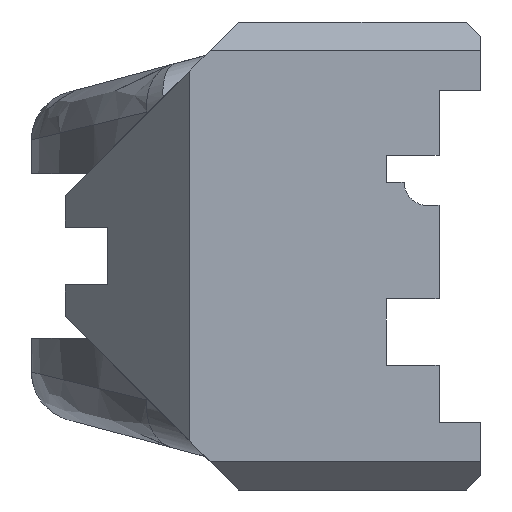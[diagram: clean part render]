
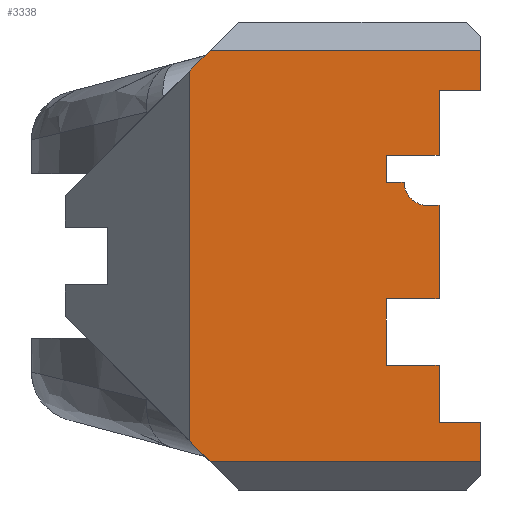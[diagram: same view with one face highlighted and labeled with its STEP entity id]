
A CAD part, left-side view. The second image highlights one B-rep face of the part: STEP entity #3338.
In plain terms, the highlighted planar face has unit normal (-1, 0, 0).
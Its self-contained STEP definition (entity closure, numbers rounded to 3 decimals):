
#82=PLANE('',#3544);
#240=FACE_OUTER_BOUND('',#420,.T.);
#420=EDGE_LOOP('',(#2469,#2470,#2471,#2472,#2473,#2474,#2475,#2476,#2477,
#2478,#2479,#2480,#2481,#2482,#2483,#2484,#2485,#2486,#2487,#2488));
#700=LINE('',#4953,#1138);
#701=LINE('',#4955,#1139);
#702=LINE('',#4957,#1140);
#703=LINE('',#4959,#1141);
#704=LINE('',#4961,#1142);
#705=LINE('',#4963,#1143);
#706=LINE('',#4965,#1144);
#707=LINE('',#4967,#1145);
#708=LINE('',#4969,#1146);
#709=LINE('',#4971,#1147);
#710=LINE('',#4973,#1148);
#711=LINE('',#4975,#1149);
#712=LINE('',#4979,#1150);
#713=LINE('',#4981,#1151);
#714=LINE('',#4983,#1152);
#715=LINE('',#4985,#1153);
#716=LINE('',#4987,#1154);
#717=LINE('',#4989,#1155);
#718=LINE('',#4990,#1156);
#1138=VECTOR('',#3966,10.);
#1139=VECTOR('',#3967,10.);
#1140=VECTOR('',#3968,10.);
#1141=VECTOR('',#3969,10.);
#1142=VECTOR('',#3970,10.);
#1143=VECTOR('',#3971,10.);
#1144=VECTOR('',#3972,10.);
#1145=VECTOR('',#3973,10.);
#1146=VECTOR('',#3974,10.);
#1147=VECTOR('',#3975,10.);
#1148=VECTOR('',#3976,10.);
#1149=VECTOR('',#3977,10.);
#1150=VECTOR('',#3980,10.);
#1151=VECTOR('',#3981,10.);
#1152=VECTOR('',#3982,10.);
#1153=VECTOR('',#3983,10.);
#1154=VECTOR('',#3984,10.);
#1155=VECTOR('',#3985,10.);
#1156=VECTOR('',#3986,10.);
#1452=CIRCLE('',#3545,1.647);
#1604=VERTEX_POINT('',#4951);
#1605=VERTEX_POINT('',#4952);
#1606=VERTEX_POINT('',#4954);
#1607=VERTEX_POINT('',#4956);
#1608=VERTEX_POINT('',#4958);
#1609=VERTEX_POINT('',#4960);
#1610=VERTEX_POINT('',#4962);
#1611=VERTEX_POINT('',#4964);
#1612=VERTEX_POINT('',#4966);
#1613=VERTEX_POINT('',#4968);
#1614=VERTEX_POINT('',#4970);
#1615=VERTEX_POINT('',#4972);
#1616=VERTEX_POINT('',#4974);
#1617=VERTEX_POINT('',#4976);
#1618=VERTEX_POINT('',#4978);
#1619=VERTEX_POINT('',#4980);
#1620=VERTEX_POINT('',#4982);
#1621=VERTEX_POINT('',#4984);
#1622=VERTEX_POINT('',#4986);
#1623=VERTEX_POINT('',#4988);
#1944=EDGE_CURVE('',#1604,#1605,#700,.T.);
#1945=EDGE_CURVE('',#1604,#1606,#701,.T.);
#1946=EDGE_CURVE('',#1607,#1606,#702,.T.);
#1947=EDGE_CURVE('',#1608,#1607,#703,.T.);
#1948=EDGE_CURVE('',#1608,#1609,#704,.T.);
#1949=EDGE_CURVE('',#1609,#1610,#705,.T.);
#1950=EDGE_CURVE('',#1610,#1611,#706,.T.);
#1951=EDGE_CURVE('',#1611,#1612,#707,.T.);
#1952=EDGE_CURVE('',#1612,#1613,#708,.T.);
#1953=EDGE_CURVE('',#1613,#1614,#709,.T.);
#1954=EDGE_CURVE('',#1614,#1615,#710,.T.);
#1955=EDGE_CURVE('',#1615,#1616,#711,.T.);
#1956=EDGE_CURVE('',#1616,#1617,#1452,.T.);
#1957=EDGE_CURVE('',#1617,#1618,#712,.T.);
#1958=EDGE_CURVE('',#1618,#1619,#713,.T.);
#1959=EDGE_CURVE('',#1619,#1620,#714,.T.);
#1960=EDGE_CURVE('',#1620,#1621,#715,.T.);
#1961=EDGE_CURVE('',#1621,#1622,#716,.T.);
#1962=EDGE_CURVE('',#1622,#1623,#717,.T.);
#1963=EDGE_CURVE('',#1605,#1623,#718,.T.);
#2469=ORIENTED_EDGE('',*,*,#1944,.F.);
#2470=ORIENTED_EDGE('',*,*,#1945,.T.);
#2471=ORIENTED_EDGE('',*,*,#1946,.F.);
#2472=ORIENTED_EDGE('',*,*,#1947,.F.);
#2473=ORIENTED_EDGE('',*,*,#1948,.T.);
#2474=ORIENTED_EDGE('',*,*,#1949,.T.);
#2475=ORIENTED_EDGE('',*,*,#1950,.T.);
#2476=ORIENTED_EDGE('',*,*,#1951,.T.);
#2477=ORIENTED_EDGE('',*,*,#1952,.T.);
#2478=ORIENTED_EDGE('',*,*,#1953,.T.);
#2479=ORIENTED_EDGE('',*,*,#1954,.T.);
#2480=ORIENTED_EDGE('',*,*,#1955,.T.);
#2481=ORIENTED_EDGE('',*,*,#1956,.T.);
#2482=ORIENTED_EDGE('',*,*,#1957,.T.);
#2483=ORIENTED_EDGE('',*,*,#1958,.T.);
#2484=ORIENTED_EDGE('',*,*,#1959,.T.);
#2485=ORIENTED_EDGE('',*,*,#1960,.T.);
#2486=ORIENTED_EDGE('',*,*,#1961,.T.);
#2487=ORIENTED_EDGE('',*,*,#1962,.T.);
#2488=ORIENTED_EDGE('',*,*,#1963,.F.);
#3338=ADVANCED_FACE('',(#240),#82,.T.);
#3544=AXIS2_PLACEMENT_3D('',#4950,#3964,#3965);
#3545=AXIS2_PLACEMENT_3D('',#4977,#3978,#3979);
#3964=DIRECTION('center_axis',(-1.,0.,0.));
#3965=DIRECTION('ref_axis',(0.,-1.,0.));
#3966=DIRECTION('',(0.,-0.707,0.707));
#3967=DIRECTION('',(0.,0.,-1.));
#3968=DIRECTION('',(0.,0.707,0.707));
#3969=DIRECTION('',(0.,1.,0.));
#3970=DIRECTION('',(0.,0.,1.));
#3971=DIRECTION('',(0.,1.,0.));
#3972=DIRECTION('',(0.,0.,1.));
#3973=DIRECTION('',(0.,1.,0.));
#3974=DIRECTION('',(0.,0.,1.));
#3975=DIRECTION('',(0.,-1.,0.));
#3976=DIRECTION('',(0.,0.,1.));
#3977=DIRECTION('',(0.,1.,0.));
#3978=DIRECTION('center_axis',(1.,0.,0.));
#3979=DIRECTION('ref_axis',(0.,1.,-0.004));
#3980=DIRECTION('',(0.,1.,0.));
#3981=DIRECTION('',(0.,0.,1.));
#3982=DIRECTION('',(0.,-1.,0.));
#3983=DIRECTION('',(0.,0.,1.));
#3984=DIRECTION('',(0.,-1.,0.));
#3985=DIRECTION('',(0.,0.,1.));
#3986=DIRECTION('',(0.,-1.,0.));
#4950=CARTESIAN_POINT('Origin',(211.305,4.902,18.207));
#4951=CARTESIAN_POINT('',(211.305,12.316,31.321));
#4952=CARTESIAN_POINT('',(211.305,10.836,32.801));
#4953=CARTESIAN_POINT('',(211.305,14.824,28.813));
#4954=CARTESIAN_POINT('',(211.305,12.316,5.092));
#4955=CARTESIAN_POINT('',(211.305,12.316,9.103));
#4956=CARTESIAN_POINT('',(211.305,10.836,3.613));
#4957=CARTESIAN_POINT('',(211.305,14.824,7.601));
#4958=CARTESIAN_POINT('',(211.305,-8.325,3.613));
#4959=CARTESIAN_POINT('',(211.305,2.913,3.613));
#4960=CARTESIAN_POINT('',(211.305,-8.325,6.39));
#4961=CARTESIAN_POINT('',(211.305,-8.325,3.613));
#4962=CARTESIAN_POINT('',(211.305,-5.385,6.39));
#4963=CARTESIAN_POINT('',(211.305,-0.242,6.39));
#4964=CARTESIAN_POINT('',(211.305,-5.385,10.447));
#4965=CARTESIAN_POINT('',(211.305,-5.385,13.479));
#4966=CARTESIAN_POINT('',(211.305,-1.65,10.447));
#4967=CARTESIAN_POINT('',(211.305,1.626,10.447));
#4968=CARTESIAN_POINT('',(211.305,-1.65,15.171));
#4969=CARTESIAN_POINT('',(211.305,-1.65,16.689));
#4970=CARTESIAN_POINT('',(211.305,-5.385,15.171));
#4971=CARTESIAN_POINT('',(211.305,-0.242,15.171));
#4972=CARTESIAN_POINT('',(211.305,-5.385,21.789));
#4973=CARTESIAN_POINT('',(211.305,-5.385,13.479));
#4974=CARTESIAN_POINT('',(211.305,-4.56,21.789));
#4975=CARTESIAN_POINT('',(211.305,0.171,21.789));
#4976=CARTESIAN_POINT('',(211.305,-2.907,23.43));
#4977=CARTESIAN_POINT('Origin',(211.305,-4.554,23.436));
#4978=CARTESIAN_POINT('',(211.305,-1.65,23.43));
#4979=CARTESIAN_POINT('',(211.305,1.626,23.43));
#4980=CARTESIAN_POINT('',(211.305,-1.65,25.345));
#4981=CARTESIAN_POINT('',(211.305,-1.65,21.776));
#4982=CARTESIAN_POINT('',(211.305,-5.385,25.345));
#4983=CARTESIAN_POINT('',(211.305,-0.242,25.345));
#4984=CARTESIAN_POINT('',(211.305,-5.385,29.923));
#4985=CARTESIAN_POINT('',(211.305,-5.385,13.479));
#4986=CARTESIAN_POINT('',(211.305,-8.325,29.923));
#4987=CARTESIAN_POINT('',(211.305,-1.985,29.923));
#4988=CARTESIAN_POINT('',(211.305,-8.325,32.801));
#4989=CARTESIAN_POINT('',(211.305,-8.325,3.613));
#4990=CARTESIAN_POINT('',(211.305,2.913,32.801));
